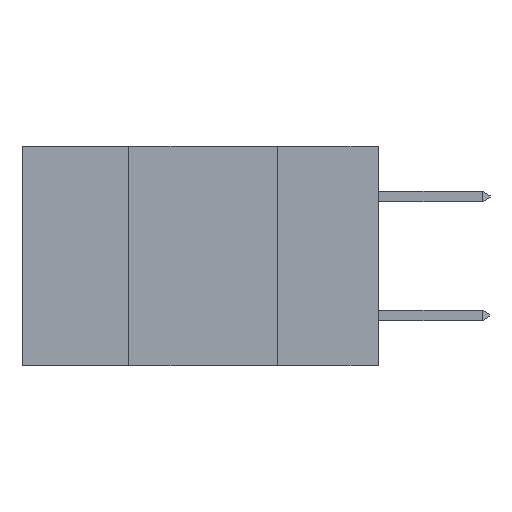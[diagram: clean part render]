
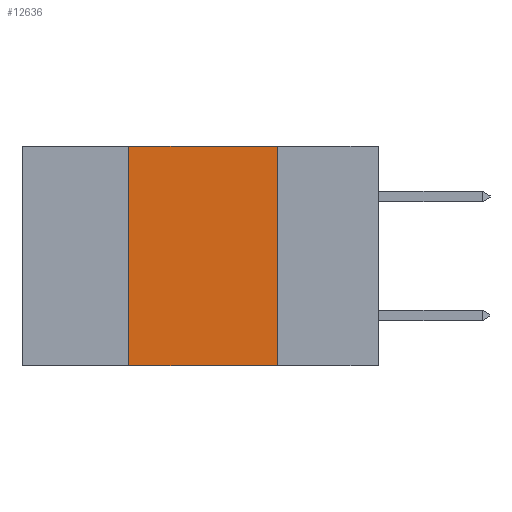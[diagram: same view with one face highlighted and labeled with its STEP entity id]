
A CAD part, left-side view. The second image highlights one B-rep face of the part: STEP entity #12636.
In plain terms, the highlighted planar face has unit normal (-1, 0, 0).
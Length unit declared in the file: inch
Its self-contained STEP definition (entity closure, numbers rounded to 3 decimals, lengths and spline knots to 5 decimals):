
#194 = CARTESIAN_POINT ( 'NONE',  ( 0., 0.42, 0. ) ) ;
#202 = CARTESIAN_POINT ( 'NONE',  ( 0., 0.17, 0. ) ) ;
#1227 = EDGE_CURVE ( 'NONE', #12431, #2295, #14852, .T. ) ;
#1913 = AXIS2_PLACEMENT_3D ( 'NONE', #10088, #5238, #13798 ) ;
#2131 = VECTOR ( 'NONE', #14812, 39.37008 ) ;
#2295 = VERTEX_POINT ( 'NONE', #10084 ) ;
#2404 = CARTESIAN_POINT ( 'NONE',  ( 0., 0.6, -0.37 ) ) ;
#2438 = CARTESIAN_POINT ( 'NONE',  ( 0., 0.6, 0. ) ) ;
#3313 = ORIENTED_EDGE ( 'NONE', *, *, #11425, .T. ) ;
#3338 = VECTOR ( 'NONE', #14716, 39.37008 ) ;
#3776 = VECTOR ( 'NONE', #15806, 39.37008 ) ;
#4034 = PLANE ( 'NONE',  #1913 ) ;
#4167 = LINE ( 'NONE', #14591, #3776 ) ;
#4201 = ORIENTED_EDGE ( 'NONE', *, *, #15528, .F. ) ;
#4845 = FACE_OUTER_BOUND ( 'NONE', #6460, .T. ) ;
#5238 = DIRECTION ( 'NONE',  ( 1., 0., 0. ) ) ;
#5981 = VERTEX_POINT ( 'NONE', #194 ) ;
#6049 = VECTOR ( 'NONE', #6195, 39.37008 ) ;
#6195 = DIRECTION ( 'NONE',  ( 0., -1., 0. ) ) ;
#6460 = EDGE_LOOP ( 'NONE', ( #7812, #4201, #7078, #3313 ) ) ;
#6997 = CARTESIAN_POINT ( 'NONE',  ( 0., 0.17, 0. ) ) ;
#7078 = ORIENTED_EDGE ( 'NONE', *, *, #14790, .F. ) ;
#7097 = VERTEX_POINT ( 'NONE', #12540 ) ;
#7812 = ORIENTED_EDGE ( 'NONE', *, *, #1227, .F. ) ;
#9681 = LINE ( 'NONE', #2438, #6049 ) ;
#10084 = CARTESIAN_POINT ( 'NONE',  ( 0., 0.17, -0.37 ) ) ;
#10088 = CARTESIAN_POINT ( 'NONE',  ( 0., 0.6, 0. ) ) ;
#11425 = EDGE_CURVE ( 'NONE', #7097, #2295, #12714, .T. ) ;
#12431 = VERTEX_POINT ( 'NONE', #6997 ) ;
#12540 = CARTESIAN_POINT ( 'NONE',  ( 0., 0.42, -0.37 ) ) ;
#12636 = ADVANCED_FACE ( 'NONE', ( #4845 ), #4034, .F. ) ;
#12714 = LINE ( 'NONE', #2404, #3338 ) ;
#13798 = DIRECTION ( 'NONE',  ( 0., 0., -1. ) ) ;
#14591 = CARTESIAN_POINT ( 'NONE',  ( 0., 0.42, 0. ) ) ;
#14716 = DIRECTION ( 'NONE',  ( 0., -1., 0. ) ) ;
#14790 = EDGE_CURVE ( 'NONE', #7097, #5981, #4167, .T. ) ;
#14812 = DIRECTION ( 'NONE',  ( 0., 0., -1. ) ) ;
#14852 = LINE ( 'NONE', #202, #2131 ) ;
#15528 = EDGE_CURVE ( 'NONE', #5981, #12431, #9681, .T. ) ;
#15806 = DIRECTION ( 'NONE',  ( 0., 0., 1. ) ) ;
